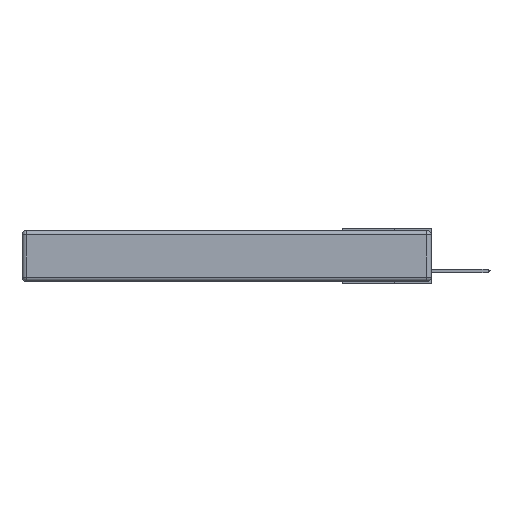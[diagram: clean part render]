
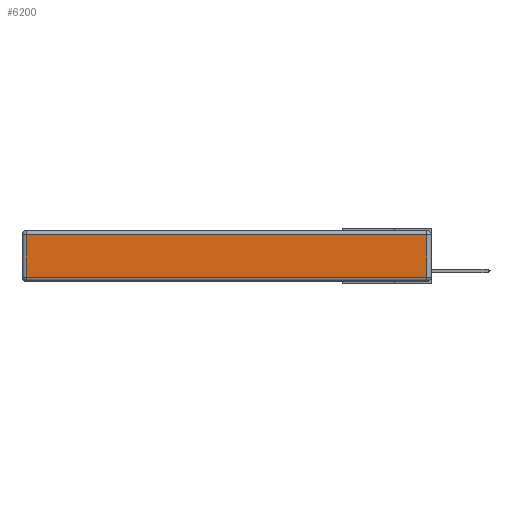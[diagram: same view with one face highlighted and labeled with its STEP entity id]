
A CAD part, left-side view. The second image highlights one B-rep face of the part: STEP entity #6200.
In plain terms, the highlighted planar face has unit normal (-1, 0, 0).
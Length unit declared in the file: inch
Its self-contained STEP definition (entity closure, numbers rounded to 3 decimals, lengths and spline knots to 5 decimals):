
#164 = VERTEX_POINT ( 'NONE', #7377 ) ;
#715 = VECTOR ( 'NONE', #10298, 39.37008 ) ;
#2153 = FACE_OUTER_BOUND ( 'NONE', #5676, .T. ) ;
#2471 = ORIENTED_EDGE ( 'NONE', *, *, #10264, .T. ) ;
#2709 = VECTOR ( 'NONE', #9144, 39.37008 ) ;
#3301 = DIRECTION ( 'NONE',  ( 0., 1., 0. ) ) ;
#3924 = CARTESIAN_POINT ( 'NONE',  ( 0., 2.72, -0.03 ) ) ;
#3938 = VERTEX_POINT ( 'NONE', #3924 ) ;
#4293 = CARTESIAN_POINT ( 'NONE',  ( 0., 2.75, -0.03 ) ) ;
#4423 = ORIENTED_EDGE ( 'NONE', *, *, #5340, .T. ) ;
#4709 = VERTEX_POINT ( 'NONE', #11100 ) ;
#5340 = EDGE_CURVE ( 'NONE', #164, #3938, #12140, .T. ) ;
#5480 = CARTESIAN_POINT ( 'NONE',  ( 0., 2.72, -0.313 ) ) ;
#5516 = DIRECTION ( 'NONE',  ( 0., 0., 1. ) ) ;
#5676 = EDGE_LOOP ( 'NONE', ( #2471, #6224, #4423, #11907 ) ) ;
#5741 = DIRECTION ( 'NONE',  ( -1., 0., 0. ) ) ;
#6139 = LINE ( 'NONE', #11971, #715 ) ;
#6200 = ADVANCED_FACE ( 'NONE', ( #2153 ), #7934, .T. ) ;
#6221 = EDGE_CURVE ( 'NONE', #3938, #11367, #6139, .T. ) ;
#6224 = ORIENTED_EDGE ( 'NONE', *, *, #7706, .T. ) ;
#7377 = CARTESIAN_POINT ( 'NONE',  ( 0., 0.03, -0.03 ) ) ;
#7706 = EDGE_CURVE ( 'NONE', #4709, #164, #11772, .T. ) ;
#7789 = DIRECTION ( 'NONE',  ( 0., 0., 1. ) ) ;
#7823 = VECTOR ( 'NONE', #5516, 39.37008 ) ;
#7934 = PLANE ( 'NONE',  #11126 ) ;
#9144 = DIRECTION ( 'NONE',  ( 0., -1., 0. ) ) ;
#10264 = EDGE_CURVE ( 'NONE', #11367, #4709, #12871, .T. ) ;
#10298 = DIRECTION ( 'NONE',  ( 0., 0., -1. ) ) ;
#11100 = CARTESIAN_POINT ( 'NONE',  ( 0., 0.03, -0.313 ) ) ;
#11126 = AXIS2_PLACEMENT_3D ( 'NONE', #11988, #5741, #7789 ) ;
#11367 = VERTEX_POINT ( 'NONE', #5480 ) ;
#11772 = LINE ( 'NONE', #12735, #7823 ) ;
#11817 = VECTOR ( 'NONE', #3301, 39.37008 ) ;
#11907 = ORIENTED_EDGE ( 'NONE', *, *, #6221, .T. ) ;
#11971 = CARTESIAN_POINT ( 'NONE',  ( 0., 2.72, -0.343 ) ) ;
#11988 = CARTESIAN_POINT ( 'NONE',  ( 0., 0., -0.343 ) ) ;
#12140 = LINE ( 'NONE', #4293, #11817 ) ;
#12735 = CARTESIAN_POINT ( 'NONE',  ( 0., 0.03, -0.343 ) ) ;
#12871 = LINE ( 'NONE', #13116, #2709 ) ;
#13116 = CARTESIAN_POINT ( 'NONE',  ( 0., 0., -0.313 ) ) ;
